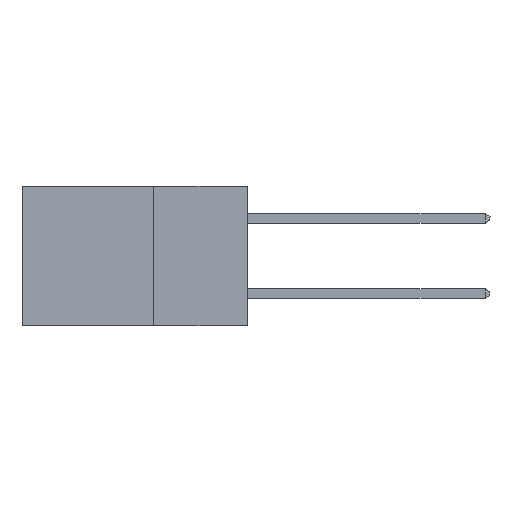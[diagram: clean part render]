
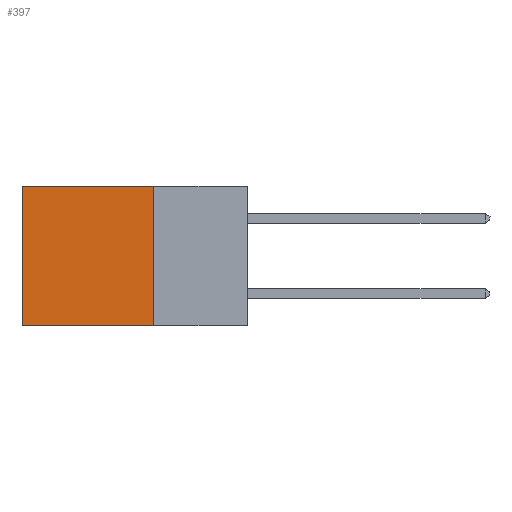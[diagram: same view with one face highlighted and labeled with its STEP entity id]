
A CAD part, left-side view. The second image highlights one B-rep face of the part: STEP entity #397.
In plain terms, the highlighted planar face has unit normal (-1, 0, 0).
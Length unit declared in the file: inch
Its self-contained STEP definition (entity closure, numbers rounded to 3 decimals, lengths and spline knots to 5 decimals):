
#397 = ADVANCED_FACE ( 'NONE', ( #1544 ), #774, .F. ) ;
#484 = VERTEX_POINT ( 'NONE', #3226 ) ;
#774 = PLANE ( 'NONE',  #818 ) ;
#818 = AXIS2_PLACEMENT_3D ( 'NONE', #8451, #5229, #9920 ) ;
#1487 = VERTEX_POINT ( 'NONE', #4410 ) ;
#1543 = EDGE_LOOP ( 'NONE', ( #2992, #6464, #3984, #8627 ) ) ;
#1544 = FACE_OUTER_BOUND ( 'NONE', #1543, .T. ) ;
#1632 = CARTESIAN_POINT ( 'NONE',  ( 0.2615, 0.25, -0.37 ) ) ;
#1712 = DIRECTION ( 'NONE',  ( 0., 1., 0. ) ) ;
#1752 = DIRECTION ( 'NONE',  ( 0., 0., -1. ) ) ;
#2303 = DIRECTION ( 'NONE',  ( 0., 1., 0. ) ) ;
#2435 = LINE ( 'NONE', #7197, #4607 ) ;
#2633 = CARTESIAN_POINT ( 'NONE',  ( 0.2615, 0.6, -0.37 ) ) ;
#2992 = ORIENTED_EDGE ( 'NONE', *, *, #6514, .T. ) ;
#3226 = CARTESIAN_POINT ( 'NONE',  ( 0.2615, 0.6, 0. ) ) ;
#3444 = LINE ( 'NONE', #2633, #6225 ) ;
#3984 = ORIENTED_EDGE ( 'NONE', *, *, #8441, .F. ) ;
#4410 = CARTESIAN_POINT ( 'NONE',  ( 0.2615, 0.25, 0. ) ) ;
#4427 = CARTESIAN_POINT ( 'NONE',  ( 0.2615, 0.25, -0.37 ) ) ;
#4563 = VECTOR ( 'NONE', #2303, 39.37008 ) ;
#4607 = VECTOR ( 'NONE', #1712, 39.37008 ) ;
#4691 = VERTEX_POINT ( 'NONE', #7817 ) ;
#5229 = DIRECTION ( 'NONE',  ( 1., 0., 0. ) ) ;
#5307 = DIRECTION ( 'NONE',  ( 0., 0., -1. ) ) ;
#5474 = LINE ( 'NONE', #1632, #4563 ) ;
#5971 = EDGE_CURVE ( 'NONE', #7318, #4691, #5474, .T. ) ;
#6082 = CARTESIAN_POINT ( 'NONE',  ( 0.2615, 0.25, -0.37 ) ) ;
#6225 = VECTOR ( 'NONE', #1752, 39.37008 ) ;
#6254 = VECTOR ( 'NONE', #5307, 39.37008 ) ;
#6464 = ORIENTED_EDGE ( 'NONE', *, *, #5971, .F. ) ;
#6514 = EDGE_CURVE ( 'NONE', #484, #4691, #3444, .T. ) ;
#6951 = LINE ( 'NONE', #6082, #6254 ) ;
#7197 = CARTESIAN_POINT ( 'NONE',  ( 0.2615, 0.25, 0. ) ) ;
#7318 = VERTEX_POINT ( 'NONE', #4427 ) ;
#7817 = CARTESIAN_POINT ( 'NONE',  ( 0.2615, 0.6, -0.37 ) ) ;
#8441 = EDGE_CURVE ( 'NONE', #1487, #7318, #6951, .T. ) ;
#8451 = CARTESIAN_POINT ( 'NONE',  ( 0.2615, 0.25, -0.37 ) ) ;
#8627 = ORIENTED_EDGE ( 'NONE', *, *, #9062, .T. ) ;
#9062 = EDGE_CURVE ( 'NONE', #1487, #484, #2435, .T. ) ;
#9920 = DIRECTION ( 'NONE',  ( 0., 0., -1. ) ) ;
